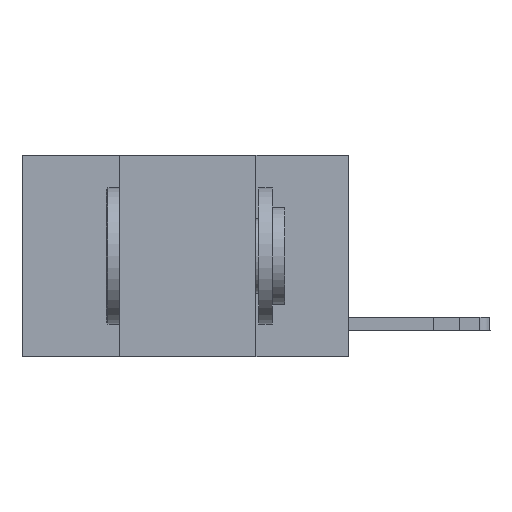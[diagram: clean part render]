
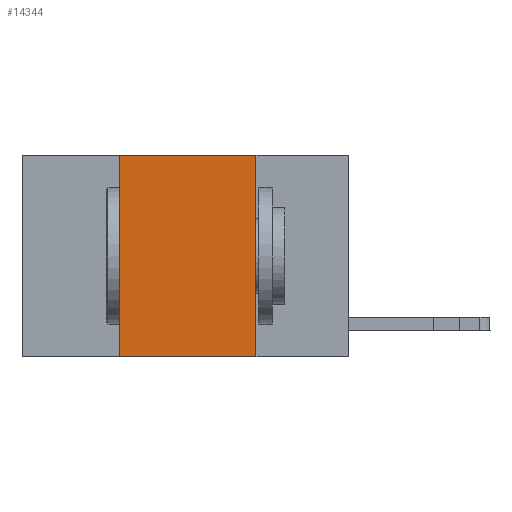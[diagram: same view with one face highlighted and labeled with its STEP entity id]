
A CAD part, left-side view. The second image highlights one B-rep face of the part: STEP entity #14344.
In plain terms, the highlighted planar face has unit normal (-1, 0, 0).
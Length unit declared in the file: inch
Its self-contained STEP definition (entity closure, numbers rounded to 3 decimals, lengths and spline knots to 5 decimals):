
#636 = CARTESIAN_POINT ( 'NONE',  ( 0., 0.17, 0. ) ) ;
#1213 = LINE ( 'NONE', #5023, #14257 ) ;
#1701 = VERTEX_POINT ( 'NONE', #7617 ) ;
#2447 = CARTESIAN_POINT ( 'NONE',  ( 0., 0.6, 0. ) ) ;
#3214 = CARTESIAN_POINT ( 'NONE',  ( 0., 0.42, 0. ) ) ;
#3910 = CARTESIAN_POINT ( 'NONE',  ( 0., 0.42, 0. ) ) ;
#5023 = CARTESIAN_POINT ( 'NONE',  ( 0., 0.6, 0. ) ) ;
#5146 = LINE ( 'NONE', #3910, #13596 ) ;
#5167 = DIRECTION ( 'NONE',  ( 1., 0., 0. ) ) ;
#5608 = VECTOR ( 'NONE', #7936, 39.37008 ) ;
#5629 = EDGE_CURVE ( 'NONE', #1701, #12658, #13984, .T. ) ;
#5708 = LINE ( 'NONE', #6526, #5608 ) ;
#5856 = EDGE_CURVE ( 'NONE', #11326, #12658, #5708, .T. ) ;
#5933 = VECTOR ( 'NONE', #7426, 39.37008 ) ;
#6255 = DIRECTION ( 'NONE',  ( 0., -1., 0. ) ) ;
#6438 = ORIENTED_EDGE ( 'NONE', *, *, #5629, .F. ) ;
#6526 = CARTESIAN_POINT ( 'NONE',  ( 0., 0.6, -0.37 ) ) ;
#6557 = EDGE_CURVE ( 'NONE', #11326, #17060, #5146, .T. ) ;
#7426 = DIRECTION ( 'NONE',  ( 0., 0., -1. ) ) ;
#7503 = ORIENTED_EDGE ( 'NONE', *, *, #5856, .T. ) ;
#7617 = CARTESIAN_POINT ( 'NONE',  ( 0., 0.17, 0. ) ) ;
#7622 = EDGE_LOOP ( 'NONE', ( #6438, #11649, #16541, #7503 ) ) ;
#7936 = DIRECTION ( 'NONE',  ( 0., -1., 0. ) ) ;
#8934 = DIRECTION ( 'NONE',  ( 0., 0., 1. ) ) ;
#10201 = EDGE_CURVE ( 'NONE', #17060, #1701, #1213, .T. ) ;
#11326 = VERTEX_POINT ( 'NONE', #13636 ) ;
#11627 = FACE_OUTER_BOUND ( 'NONE', #7622, .T. ) ;
#11649 = ORIENTED_EDGE ( 'NONE', *, *, #10201, .F. ) ;
#12658 = VERTEX_POINT ( 'NONE', #16303 ) ;
#13596 = VECTOR ( 'NONE', #8934, 39.37008 ) ;
#13636 = CARTESIAN_POINT ( 'NONE',  ( 0., 0.42, -0.37 ) ) ;
#13984 = LINE ( 'NONE', #636, #5933 ) ;
#14046 = AXIS2_PLACEMENT_3D ( 'NONE', #2447, #5167, #16130 ) ;
#14257 = VECTOR ( 'NONE', #6255, 39.37008 ) ;
#14344 = ADVANCED_FACE ( 'NONE', ( #11627 ), #17296, .F. ) ;
#16130 = DIRECTION ( 'NONE',  ( 0., 0., -1. ) ) ;
#16303 = CARTESIAN_POINT ( 'NONE',  ( 0., 0.17, -0.37 ) ) ;
#16541 = ORIENTED_EDGE ( 'NONE', *, *, #6557, .F. ) ;
#17060 = VERTEX_POINT ( 'NONE', #3214 ) ;
#17296 = PLANE ( 'NONE',  #14046 ) ;
